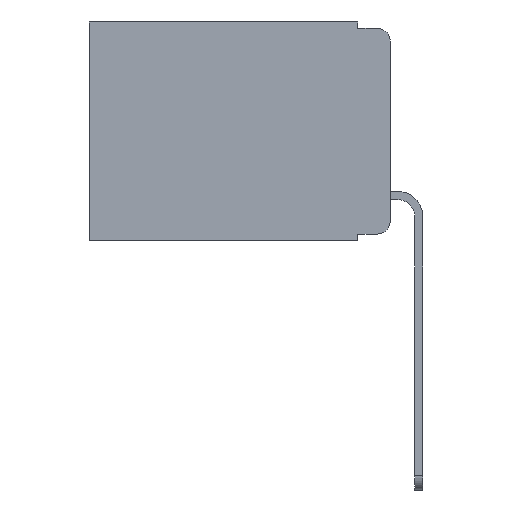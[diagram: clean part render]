
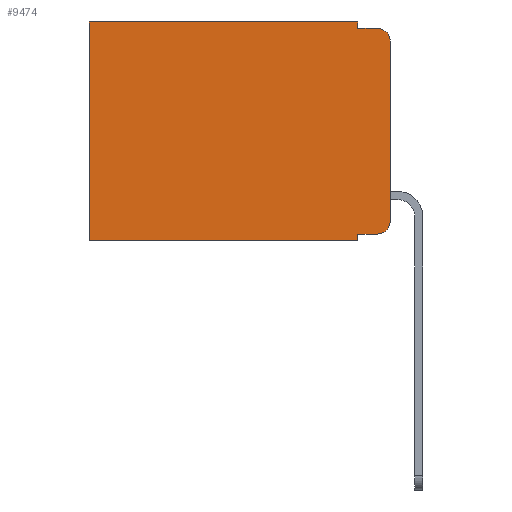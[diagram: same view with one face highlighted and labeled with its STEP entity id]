
A CAD part, left-side view. The second image highlights one B-rep face of the part: STEP entity #9474.
In plain terms, the highlighted planar face has unit normal (-1, 0, 0).
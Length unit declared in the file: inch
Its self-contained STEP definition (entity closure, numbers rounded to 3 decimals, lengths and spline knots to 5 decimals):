
#59 = LINE ( 'NONE', #867, #8309 ) ;
#497 = VERTEX_POINT ( 'NONE', #6959 ) ;
#616 = LINE ( 'NONE', #3987, #8713 ) ;
#726 = CARTESIAN_POINT ( 'NONE',  ( 0.298, 0.051, 0. ) ) ;
#827 = DIRECTION ( 'NONE',  ( 0., 0., -1. ) ) ;
#867 = CARTESIAN_POINT ( 'NONE',  ( 0.298, 0.051, -0.333 ) ) ;
#1242 = EDGE_CURVE ( 'NONE', #2879, #3369, #5634, .T. ) ;
#1391 = LINE ( 'NONE', #7916, #7175 ) ;
#1399 = ORIENTED_EDGE ( 'NONE', *, *, #1242, .F. ) ;
#1492 = ORIENTED_EDGE ( 'NONE', *, *, #3710, .T. ) ;
#1501 = ORIENTED_EDGE ( 'NONE', *, *, #5756, .T. ) ;
#1516 = ORIENTED_EDGE ( 'NONE', *, *, #6517, .F. ) ;
#1688 = VERTEX_POINT ( 'NONE', #2842 ) ;
#1692 = CIRCLE ( 'NONE', #9051, 0.02 ) ;
#1749 = ORIENTED_EDGE ( 'NONE', *, *, #6467, .F. ) ;
#1881 = DIRECTION ( 'NONE',  ( 0., 1., 0. ) ) ;
#1893 = ORIENTED_EDGE ( 'NONE', *, *, #5928, .F. ) ;
#2135 = CARTESIAN_POINT ( 'NONE',  ( 0.298, 0.02, -0.313 ) ) ;
#2140 = DIRECTION ( 'NONE',  ( 0., 0., -1. ) ) ;
#2143 = VECTOR ( 'NONE', #8318, 39.37008 ) ;
#2146 = DIRECTION ( 'NONE',  ( -1., 0., 0. ) ) ;
#2156 = CARTESIAN_POINT ( 'NONE',  ( 0.298, 0.02, -0.03 ) ) ;
#2188 = ORIENTED_EDGE ( 'NONE', *, *, #6129, .T. ) ;
#2280 = VERTEX_POINT ( 'NONE', #8338 ) ;
#2842 = CARTESIAN_POINT ( 'NONE',  ( 0.298, 0.02, -0.333 ) ) ;
#2879 = VERTEX_POINT ( 'NONE', #6969 ) ;
#2985 = DIRECTION ( 'NONE',  ( 0., 0., -1. ) ) ;
#3291 = CARTESIAN_POINT ( 'NONE',  ( 0.298, 0., 0. ) ) ;
#3369 = VERTEX_POINT ( 'NONE', #8404 ) ;
#3445 = CARTESIAN_POINT ( 'NONE',  ( 0.298, 0., 0. ) ) ;
#3511 = DIRECTION ( 'NONE',  ( 0., 0., -1. ) ) ;
#3710 = EDGE_CURVE ( 'NONE', #2280, #3369, #616, .T. ) ;
#3987 = CARTESIAN_POINT ( 'NONE',  ( 0.298, 0.473, 0. ) ) ;
#4121 = CARTESIAN_POINT ( 'NONE',  ( 0.298, 0.051, 0. ) ) ;
#4219 = LINE ( 'NONE', #3291, #5943 ) ;
#4253 = EDGE_LOOP ( 'NONE', ( #1893, #2188, #1749, #1516, #1501, #1492, #1399, #9682, #8231, #5265 ) ) ;
#4266 = CARTESIAN_POINT ( 'NONE',  ( 0.298, 0., -0.313 ) ) ;
#4274 = DIRECTION ( 'NONE',  ( 0., 0., -1. ) ) ;
#4275 = VERTEX_POINT ( 'NONE', #6541 ) ;
#4293 = VERTEX_POINT ( 'NONE', #8272 ) ;
#4655 = FACE_OUTER_BOUND ( 'NONE', #4253, .T. ) ;
#5089 = AXIS2_PLACEMENT_3D ( 'NONE', #3445, #8772, #4274 ) ;
#5265 = ORIENTED_EDGE ( 'NONE', *, *, #8523, .T. ) ;
#5342 = VERTEX_POINT ( 'NONE', #4266 ) ;
#5634 = LINE ( 'NONE', #5949, #9385 ) ;
#5756 = EDGE_CURVE ( 'NONE', #6434, #2280, #1391, .T. ) ;
#5882 = CARTESIAN_POINT ( 'NONE',  ( 0.298, 0.051, -0.01 ) ) ;
#5928 = EDGE_CURVE ( 'NONE', #497, #5342, #4219, .T. ) ;
#5943 = VECTOR ( 'NONE', #9444, 39.37008 ) ;
#5949 = CARTESIAN_POINT ( 'NONE',  ( 0.298, 0., -0.343 ) ) ;
#6129 = EDGE_CURVE ( 'NONE', #497, #4275, #6559, .T. ) ;
#6215 = DIRECTION ( 'NONE',  ( 0., 1., 0. ) ) ;
#6300 = LINE ( 'NONE', #7954, #2143 ) ;
#6412 = DIRECTION ( 'NONE',  ( 0., -1., 0. ) ) ;
#6434 = VERTEX_POINT ( 'NONE', #726 ) ;
#6467 = EDGE_CURVE ( 'NONE', #7616, #4275, #6300, .T. ) ;
#6517 = EDGE_CURVE ( 'NONE', #6434, #7616, #8136, .T. ) ;
#6541 = CARTESIAN_POINT ( 'NONE',  ( 0.298, 0.02, -0.01 ) ) ;
#6559 = CIRCLE ( 'NONE', #8334, 0.02 ) ;
#6730 = LINE ( 'NONE', #4121, #8539 ) ;
#6959 = CARTESIAN_POINT ( 'NONE',  ( 0.298, 0., -0.03 ) ) ;
#6969 = CARTESIAN_POINT ( 'NONE',  ( 0.298, 0.051, -0.343 ) ) ;
#7175 = VECTOR ( 'NONE', #1881, 39.37008 ) ;
#7616 = VERTEX_POINT ( 'NONE', #5882 ) ;
#7618 = DIRECTION ( 'NONE',  ( -1., 0., 0. ) ) ;
#7916 = CARTESIAN_POINT ( 'NONE',  ( 0.298, 0., 0. ) ) ;
#7954 = CARTESIAN_POINT ( 'NONE',  ( 0.298, 0.051, -0.01 ) ) ;
#8069 = PLANE ( 'NONE',  #5089 ) ;
#8136 = LINE ( 'NONE', #8301, #9587 ) ;
#8231 = ORIENTED_EDGE ( 'NONE', *, *, #8790, .T. ) ;
#8272 = CARTESIAN_POINT ( 'NONE',  ( 0.298, 0.051, -0.333 ) ) ;
#8301 = CARTESIAN_POINT ( 'NONE',  ( 0.298, 0.051, 0. ) ) ;
#8309 = VECTOR ( 'NONE', #6412, 39.37008 ) ;
#8318 = DIRECTION ( 'NONE',  ( 0., -1., 0. ) ) ;
#8334 = AXIS2_PLACEMENT_3D ( 'NONE', #2156, #2146, #2140 ) ;
#8338 = CARTESIAN_POINT ( 'NONE',  ( 0.298, 0.473, 0. ) ) ;
#8404 = CARTESIAN_POINT ( 'NONE',  ( 0.298, 0.473, -0.343 ) ) ;
#8523 = EDGE_CURVE ( 'NONE', #1688, #5342, #1692, .T. ) ;
#8539 = VECTOR ( 'NONE', #827, 39.37008 ) ;
#8713 = VECTOR ( 'NONE', #3511, 39.37008 ) ;
#8740 = EDGE_CURVE ( 'NONE', #4293, #2879, #6730, .T. ) ;
#8772 = DIRECTION ( 'NONE',  ( 1., 0., 0. ) ) ;
#8790 = EDGE_CURVE ( 'NONE', #4293, #1688, #59, .T. ) ;
#9051 = AXIS2_PLACEMENT_3D ( 'NONE', #2135, #7618, #2985 ) ;
#9385 = VECTOR ( 'NONE', #6215, 39.37008 ) ;
#9444 = DIRECTION ( 'NONE',  ( 0., 0., -1. ) ) ;
#9474 = ADVANCED_FACE ( 'NONE', ( #4655 ), #8069, .F. ) ;
#9587 = VECTOR ( 'NONE', #9894, 39.37008 ) ;
#9682 = ORIENTED_EDGE ( 'NONE', *, *, #8740, .F. ) ;
#9894 = DIRECTION ( 'NONE',  ( 0., 0., -1. ) ) ;
